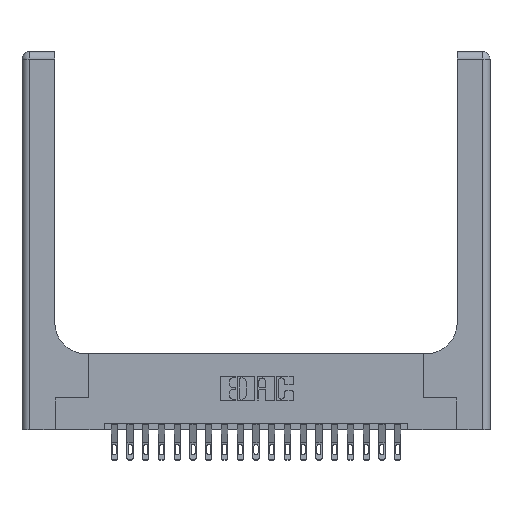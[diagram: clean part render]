
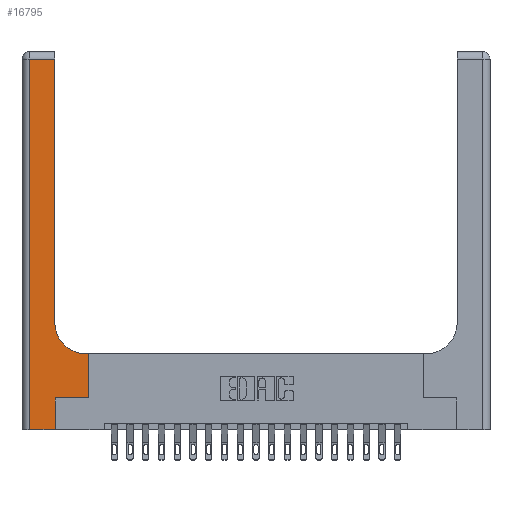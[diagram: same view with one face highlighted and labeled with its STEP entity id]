
A CAD part, top view. The second image highlights one B-rep face of the part: STEP entity #16795.
In plain terms, the highlighted planar face has unit normal (0, 0, 1).
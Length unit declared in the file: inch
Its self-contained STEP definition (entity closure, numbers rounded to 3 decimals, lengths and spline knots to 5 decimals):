
#220 = VECTOR ( 'NONE', #17694, 39.37008 ) ;
#1034 = ORIENTED_EDGE ( 'NONE', *, *, #21003, .T. ) ;
#1286 = CARTESIAN_POINT ( 'NONE',  ( 0.06, 3., 0.37 ) ) ;
#1790 = EDGE_CURVE ( 'NONE', #10984, #20796, #18435, .T. ) ;
#1947 = CARTESIAN_POINT ( 'NONE',  ( 0.06, 0., 0.37 ) ) ;
#2965 = CARTESIAN_POINT ( 'NONE',  ( 0.265, 0.25, 0.37 ) ) ;
#4026 = CARTESIAN_POINT ( 'NONE',  ( 0.265, 0., 0.37 ) ) ;
#4632 = EDGE_LOOP ( 'NONE', ( #15497, #1034, #19154, #6815, #6282, #6241, #19794, #8560, #12209 ) ) ;
#5083 = CIRCLE ( 'NONE', #5841, 0.25 ) ;
#5248 = CARTESIAN_POINT ( 'NONE',  ( 0.06, 2.94, 0.37 ) ) ;
#5588 = EDGE_CURVE ( 'NONE', #12101, #9866, #10195, .T. ) ;
#5841 = AXIS2_PLACEMENT_3D ( 'NONE', #9348, #17558, #20810 ) ;
#5949 = DIRECTION ( 'NONE',  ( -1., 0., 0. ) ) ;
#6241 = ORIENTED_EDGE ( 'NONE', *, *, #19449, .T. ) ;
#6272 = EDGE_CURVE ( 'NONE', #13133, #12101, #5083, .T. ) ;
#6282 = ORIENTED_EDGE ( 'NONE', *, *, #1790, .T. ) ;
#6815 = ORIENTED_EDGE ( 'NONE', *, *, #14433, .T. ) ;
#7511 = EDGE_CURVE ( 'NONE', #18604, #13133, #16245, .T. ) ;
#8560 = ORIENTED_EDGE ( 'NONE', *, *, #7511, .T. ) ;
#8843 = CARTESIAN_POINT ( 'NONE',  ( 0.26, 0.85, 0.37 ) ) ;
#8983 = EDGE_CURVE ( 'NONE', #17237, #17337, #18603, .T. ) ;
#9244 = CARTESIAN_POINT ( 'NONE',  ( 0., 2.94, 0.37 ) ) ;
#9348 = CARTESIAN_POINT ( 'NONE',  ( 0.51, 0.85, 0.37 ) ) ;
#9449 = DIRECTION ( 'NONE',  ( 1., 0., 0. ) ) ;
#9746 = VECTOR ( 'NONE', #14556, 39.37008 ) ;
#9755 = DIRECTION ( 'NONE',  ( 0., 1., 0. ) ) ;
#9866 = VERTEX_POINT ( 'NONE', #19107 ) ;
#10195 = LINE ( 'NONE', #13093, #10709 ) ;
#10709 = VECTOR ( 'NONE', #9755, 39.37008 ) ;
#10984 = VERTEX_POINT ( 'NONE', #4026 ) ;
#11077 = DIRECTION ( 'NONE',  ( 0., -1., 0. ) ) ;
#11345 = DIRECTION ( 'NONE',  ( 1., 0., 0. ) ) ;
#11613 = DIRECTION ( 'NONE',  ( 0., 0., -1. ) ) ;
#11781 = CARTESIAN_POINT ( 'NONE',  ( 0.265, 0., 0.37 ) ) ;
#11932 = CARTESIAN_POINT ( 'NONE',  ( 0.528, 0.25, 0.37 ) ) ;
#12101 = VERTEX_POINT ( 'NONE', #8843 ) ;
#12209 = ORIENTED_EDGE ( 'NONE', *, *, #6272, .T. ) ;
#12524 = CARTESIAN_POINT ( 'NONE',  ( 0.528, 0.25, 0.37 ) ) ;
#13002 = CARTESIAN_POINT ( 'NONE',  ( 0.265, 0.25, 0.37 ) ) ;
#13085 = VECTOR ( 'NONE', #9449, 39.37008 ) ;
#13093 = CARTESIAN_POINT ( 'NONE',  ( 0.26, 3., 0.37 ) ) ;
#13106 = PLANE ( 'NONE',  #16849 ) ;
#13133 = VERTEX_POINT ( 'NONE', #17285 ) ;
#13175 = CARTESIAN_POINT ( 'NONE',  ( 0., 3., 0.37 ) ) ;
#13251 = DIRECTION ( 'NONE',  ( -1., 0., 0. ) ) ;
#14433 = EDGE_CURVE ( 'NONE', #17337, #10984, #16095, .T. ) ;
#14556 = DIRECTION ( 'NONE',  ( 0., 1., 0. ) ) ;
#14569 = CARTESIAN_POINT ( 'NONE',  ( 0.26, 0.6, 0.37 ) ) ;
#15497 = ORIENTED_EDGE ( 'NONE', *, *, #5588, .T. ) ;
#15794 = VECTOR ( 'NONE', #11077, 39.37008 ) ;
#15937 = VECTOR ( 'NONE', #16394, 39.37008 ) ;
#16095 = LINE ( 'NONE', #20618, #17616 ) ;
#16245 = LINE ( 'NONE', #14569, #220 ) ;
#16307 = VERTEX_POINT ( 'NONE', #11932 ) ;
#16394 = DIRECTION ( 'NONE',  ( 0., 1., 0. ) ) ;
#16795 = ADVANCED_FACE ( 'NONE', ( #18512 ), #13106, .F. ) ;
#16849 = AXIS2_PLACEMENT_3D ( 'NONE', #13175, #11613, #13251 ) ;
#17237 = VERTEX_POINT ( 'NONE', #5248 ) ;
#17285 = CARTESIAN_POINT ( 'NONE',  ( 0.51, 0.6, 0.37 ) ) ;
#17330 = LINE ( 'NONE', #9244, #19366 ) ;
#17337 = VERTEX_POINT ( 'NONE', #1947 ) ;
#17558 = DIRECTION ( 'NONE',  ( 0., 0., -1. ) ) ;
#17616 = VECTOR ( 'NONE', #11345, 39.37008 ) ;
#17694 = DIRECTION ( 'NONE',  ( -1., 0., 0. ) ) ;
#18207 = CARTESIAN_POINT ( 'NONE',  ( 0.528, 0.6, 0.37 ) ) ;
#18435 = LINE ( 'NONE', #11781, #15937 ) ;
#18512 = FACE_OUTER_BOUND ( 'NONE', #4632, .T. ) ;
#18603 = LINE ( 'NONE', #1286, #15794 ) ;
#18604 = VERTEX_POINT ( 'NONE', #18207 ) ;
#19107 = CARTESIAN_POINT ( 'NONE',  ( 0.26, 2.94, 0.37 ) ) ;
#19149 = LINE ( 'NONE', #12524, #9746 ) ;
#19154 = ORIENTED_EDGE ( 'NONE', *, *, #8983, .T. ) ;
#19366 = VECTOR ( 'NONE', #5949, 39.37008 ) ;
#19449 = EDGE_CURVE ( 'NONE', #20796, #16307, #20940, .T. ) ;
#19794 = ORIENTED_EDGE ( 'NONE', *, *, #20566, .T. ) ;
#20566 = EDGE_CURVE ( 'NONE', #16307, #18604, #19149, .T. ) ;
#20618 = CARTESIAN_POINT ( 'NONE',  ( 0., 0., 0.37 ) ) ;
#20796 = VERTEX_POINT ( 'NONE', #13002 ) ;
#20810 = DIRECTION ( 'NONE',  ( 1., 0., 0. ) ) ;
#20940 = LINE ( 'NONE', #2965, #13085 ) ;
#21003 = EDGE_CURVE ( 'NONE', #9866, #17237, #17330, .T. ) ;
